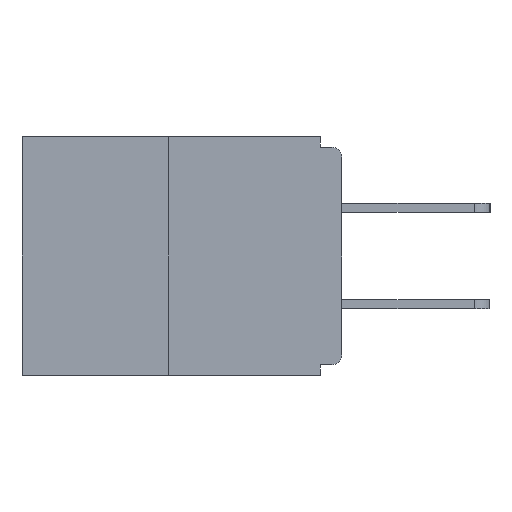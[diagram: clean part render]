
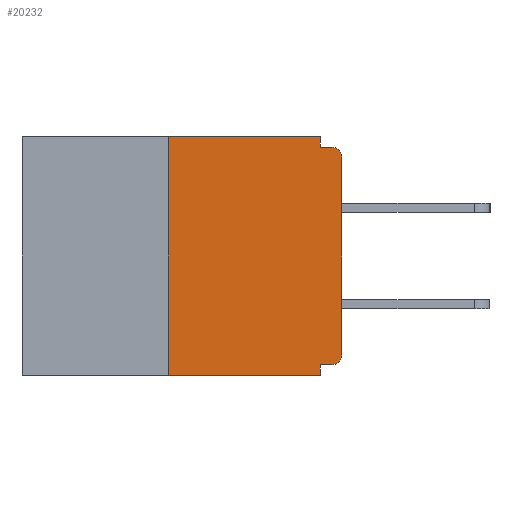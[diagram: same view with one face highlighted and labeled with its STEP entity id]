
A CAD part, left-side view. The second image highlights one B-rep face of the part: STEP entity #20232.
In plain terms, the highlighted planar face has unit normal (-1, 0, 0).
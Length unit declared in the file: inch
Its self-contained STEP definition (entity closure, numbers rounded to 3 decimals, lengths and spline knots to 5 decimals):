
#169 = VERTEX_POINT ( 'NONE', #813 ) ;
#181 = DIRECTION ( 'NONE',  ( 0., 0., -1. ) ) ;
#750 = LINE ( 'NONE', #5963, #14869 ) ;
#813 = CARTESIAN_POINT ( 'NONE',  ( 0., 0.031, -0.343 ) ) ;
#855 = VERTEX_POINT ( 'NONE', #11574 ) ;
#858 = EDGE_CURVE ( 'NONE', #18321, #11315, #1644, .T. ) ;
#966 = EDGE_CURVE ( 'NONE', #20010, #14482, #16368, .T. ) ;
#1014 = VERTEX_POINT ( 'NONE', #5311 ) ;
#1188 = ORIENTED_EDGE ( 'NONE', *, *, #11414, .T. ) ;
#1265 = VECTOR ( 'NONE', #12197, 39.37008 ) ;
#1644 = LINE ( 'NONE', #13143, #13103 ) ;
#1839 = ORIENTED_EDGE ( 'NONE', *, *, #966, .F. ) ;
#2683 = CARTESIAN_POINT ( 'NONE',  ( 0., 0.46, -0.343 ) ) ;
#3786 = CIRCLE ( 'NONE', #15566, 0.015 ) ;
#3940 = LINE ( 'NONE', #15530, #18865 ) ;
#4353 = LINE ( 'NONE', #20254, #11565 ) ;
#4694 = DIRECTION ( 'NONE',  ( 0., -1., 0. ) ) ;
#4799 = VECTOR ( 'NONE', #10598, 39.37008 ) ;
#4875 = CARTESIAN_POINT ( 'NONE',  ( 0., 0.25, -0.343 ) ) ;
#4907 = DIRECTION ( 'NONE',  ( 1., 0., 0. ) ) ;
#4985 = ORIENTED_EDGE ( 'NONE', *, *, #18491, .F. ) ;
#5311 = CARTESIAN_POINT ( 'NONE',  ( 0., 0., -0.03 ) ) ;
#5440 = DIRECTION ( 'NONE',  ( -1., 0., 0. ) ) ;
#5752 = EDGE_CURVE ( 'NONE', #1014, #855, #3786, .T. ) ;
#5963 = CARTESIAN_POINT ( 'NONE',  ( 0., 0.46, 0. ) ) ;
#6238 = ORIENTED_EDGE ( 'NONE', *, *, #7883, .T. ) ;
#6403 = ORIENTED_EDGE ( 'NONE', *, *, #7696, .T. ) ;
#6814 = PLANE ( 'NONE',  #17560 ) ;
#6852 = ORIENTED_EDGE ( 'NONE', *, *, #20042, .F. ) ;
#7180 = EDGE_LOOP ( 'NONE', ( #6852, #15912, #6238, #4985, #1839, #6403, #1188, #12221, #10258, #13938 ) ) ;
#7245 = CARTESIAN_POINT ( 'NONE',  ( 0., 0.031, -0.328 ) ) ;
#7696 = EDGE_CURVE ( 'NONE', #20010, #9207, #10009, .T. ) ;
#7883 = EDGE_CURVE ( 'NONE', #17848, #169, #12511, .T. ) ;
#8609 = DIRECTION ( 'NONE',  ( 0., 1., 0. ) ) ;
#8914 = DIRECTION ( 'NONE',  ( 0., -1., 0. ) ) ;
#9207 = VERTEX_POINT ( 'NONE', #13295 ) ;
#10009 = CIRCLE ( 'NONE', #17386, 0.015 ) ;
#10258 = ORIENTED_EDGE ( 'NONE', *, *, #18806, .F. ) ;
#10598 = DIRECTION ( 'NONE',  ( 0., 0., 1. ) ) ;
#11140 = LINE ( 'NONE', #16059, #11862 ) ;
#11315 = VERTEX_POINT ( 'NONE', #19654 ) ;
#11414 = EDGE_CURVE ( 'NONE', #9207, #1014, #4353, .T. ) ;
#11521 = EDGE_CURVE ( 'NONE', #17848, #15461, #15529, .T. ) ;
#11565 = VECTOR ( 'NONE', #20462, 39.37008 ) ;
#11574 = CARTESIAN_POINT ( 'NONE',  ( 0., 0.015, -0.015 ) ) ;
#11587 = CARTESIAN_POINT ( 'NONE',  ( 0., 0.015, -0.313 ) ) ;
#11862 = VECTOR ( 'NONE', #17646, 39.37008 ) ;
#12197 = DIRECTION ( 'NONE',  ( 0., -1., 0. ) ) ;
#12221 = ORIENTED_EDGE ( 'NONE', *, *, #5752, .T. ) ;
#12511 = LINE ( 'NONE', #2683, #1265 ) ;
#13103 = VECTOR ( 'NONE', #14707, 39.37008 ) ;
#13143 = CARTESIAN_POINT ( 'NONE',  ( 0., 0.031, 0. ) ) ;
#13295 = CARTESIAN_POINT ( 'NONE',  ( 0., 0., -0.313 ) ) ;
#13938 = ORIENTED_EDGE ( 'NONE', *, *, #858, .F. ) ;
#14482 = VERTEX_POINT ( 'NONE', #7245 ) ;
#14707 = DIRECTION ( 'NONE',  ( 0., 0., -1. ) ) ;
#14869 = VECTOR ( 'NONE', #4694, 39.37008 ) ;
#15026 = DIRECTION ( 'NONE',  ( 0., 0., -1. ) ) ;
#15066 = CARTESIAN_POINT ( 'NONE',  ( 0., 0.031, 0. ) ) ;
#15115 = CARTESIAN_POINT ( 'NONE',  ( 0., 0., -0.328 ) ) ;
#15461 = VERTEX_POINT ( 'NONE', #19257 ) ;
#15529 = LINE ( 'NONE', #20358, #4799 ) ;
#15530 = CARTESIAN_POINT ( 'NONE',  ( 0., 0., -0.015 ) ) ;
#15566 = AXIS2_PLACEMENT_3D ( 'NONE', #17330, #18601, #20288 ) ;
#15912 = ORIENTED_EDGE ( 'NONE', *, *, #11521, .F. ) ;
#16059 = CARTESIAN_POINT ( 'NONE',  ( 0., 0.031, -0.343 ) ) ;
#16067 = FACE_OUTER_BOUND ( 'NONE', #7180, .T. ) ;
#16362 = VECTOR ( 'NONE', #8609, 39.37008 ) ;
#16368 = LINE ( 'NONE', #15115, #16362 ) ;
#17330 = CARTESIAN_POINT ( 'NONE',  ( 0., 0.015, -0.03 ) ) ;
#17386 = AXIS2_PLACEMENT_3D ( 'NONE', #11587, #5440, #15026 ) ;
#17560 = AXIS2_PLACEMENT_3D ( 'NONE', #19663, #4907, #181 ) ;
#17646 = DIRECTION ( 'NONE',  ( 0., 0., -1. ) ) ;
#17848 = VERTEX_POINT ( 'NONE', #4875 ) ;
#18114 = CARTESIAN_POINT ( 'NONE',  ( 0., 0.015, -0.328 ) ) ;
#18321 = VERTEX_POINT ( 'NONE', #15066 ) ;
#18491 = EDGE_CURVE ( 'NONE', #14482, #169, #11140, .T. ) ;
#18601 = DIRECTION ( 'NONE',  ( -1., 0., 0. ) ) ;
#18806 = EDGE_CURVE ( 'NONE', #11315, #855, #3940, .T. ) ;
#18865 = VECTOR ( 'NONE', #8914, 39.37008 ) ;
#19257 = CARTESIAN_POINT ( 'NONE',  ( 0., 0.25, 0. ) ) ;
#19654 = CARTESIAN_POINT ( 'NONE',  ( 0., 0.031, -0.015 ) ) ;
#19663 = CARTESIAN_POINT ( 'NONE',  ( 0., 0.46, 0. ) ) ;
#20010 = VERTEX_POINT ( 'NONE', #18114 ) ;
#20042 = EDGE_CURVE ( 'NONE', #15461, #18321, #750, .T. ) ;
#20232 = ADVANCED_FACE ( 'NONE', ( #16067 ), #6814, .F. ) ;
#20254 = CARTESIAN_POINT ( 'NONE',  ( 0., 0., 0. ) ) ;
#20288 = DIRECTION ( 'NONE',  ( 0., 0., -1. ) ) ;
#20358 = CARTESIAN_POINT ( 'NONE',  ( 0., 0.25, 0. ) ) ;
#20462 = DIRECTION ( 'NONE',  ( 0., 0., 1. ) ) ;
